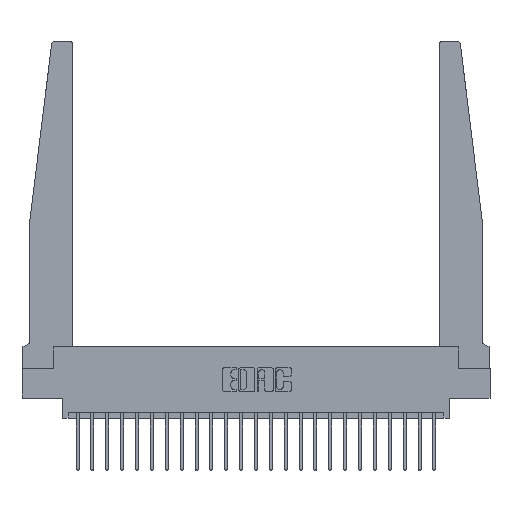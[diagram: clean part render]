
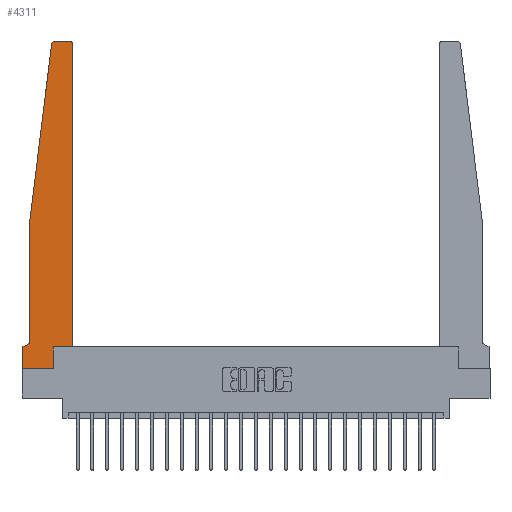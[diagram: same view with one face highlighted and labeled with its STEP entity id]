
A CAD part, top view. The second image highlights one B-rep face of the part: STEP entity #4311.
In plain terms, the highlighted planar face has unit normal (0, 0, 1).
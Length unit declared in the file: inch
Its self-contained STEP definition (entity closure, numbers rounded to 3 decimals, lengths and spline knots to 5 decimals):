
#59 = VERTEX_POINT ( 'NONE', #22046 ) ;
#147 = CARTESIAN_POINT ( 'NONE',  ( 0., 0., 0.37 ) ) ;
#385 = VECTOR ( 'NONE', #1121, 39.37008 ) ;
#510 = CARTESIAN_POINT ( 'NONE',  ( 0., 0.1875, 0.37 ) ) ;
#594 = CIRCLE ( 'NONE', #5047, 0.05 ) ;
#665 = CARTESIAN_POINT ( 'NONE',  ( 0.425, 0.18, 0.37 ) ) ;
#857 = CARTESIAN_POINT ( 'NONE',  ( 0., 0., 0.37 ) ) ;
#860 = LINE ( 'NONE', #13269, #14882 ) ;
#874 = AXIS2_PLACEMENT_3D ( 'NONE', #9341, #22089, #11198 ) ;
#892 = CARTESIAN_POINT ( 'NONE',  ( 0.24675, 2.72367, 0.37 ) ) ;
#988 = CARTESIAN_POINT ( 'NONE',  ( 0.25, 2.75, 0.37 ) ) ;
#1107 = DIRECTION ( 'NONE',  ( 0., 0., -1. ) ) ;
#1121 = DIRECTION ( 'NONE',  ( -1., 0., 0. ) ) ;
#1169 = DIRECTION ( 'NONE',  ( -0.122, -0.992, 0. ) ) ;
#2111 = EDGE_CURVE ( 'NONE', #6656, #59, #3612, .T. ) ;
#2179 = ORIENTED_EDGE ( 'NONE', *, *, #13527, .T. ) ;
#2462 = DIRECTION ( 'NONE',  ( 1., 0., 0. ) ) ;
#2829 = ORIENTED_EDGE ( 'NONE', *, *, #20193, .T. ) ;
#3406 = DIRECTION ( 'NONE',  ( 0., -1., 0. ) ) ;
#3612 = LINE ( 'NONE', #16881, #12784 ) ;
#3784 = CARTESIAN_POINT ( 'NONE',  ( 0.425, 2.72, 0.37 ) ) ;
#4311 = ADVANCED_FACE ( 'NONE', ( #18955 ), #8320, .T. ) ;
#4399 = LINE ( 'NONE', #10229, #13572 ) ;
#4534 = LINE ( 'NONE', #665, #18586 ) ;
#4621 = VERTEX_POINT ( 'NONE', #9284 ) ;
#4689 = CARTESIAN_POINT ( 'NONE',  ( 0., 0.1875, 0.37 ) ) ;
#4871 = VERTEX_POINT ( 'NONE', #857 ) ;
#4925 = LINE ( 'NONE', #21740, #14113 ) ;
#5047 = AXIS2_PLACEMENT_3D ( 'NONE', #12007, #1107, #13897 ) ;
#5271 = VERTEX_POINT ( 'NONE', #7310 ) ;
#5680 = DIRECTION ( 'NONE',  ( 1., 0., 0. ) ) ;
#5751 = LINE ( 'NONE', #10177, #385 ) ;
#5946 = DIRECTION ( 'NONE',  ( 0., 1., 0. ) ) ;
#6105 = VERTEX_POINT ( 'NONE', #7841 ) ;
#6249 = EDGE_CURVE ( 'NONE', #14112, #13678, #5751, .T. ) ;
#6656 = VERTEX_POINT ( 'NONE', #20391 ) ;
#7025 = LINE ( 'NONE', #147, #21035 ) ;
#7199 = DIRECTION ( 'NONE',  ( 0., 1., 0. ) ) ;
#7310 = CARTESIAN_POINT ( 'NONE',  ( 0.2605, 0.18, 0.37 ) ) ;
#7724 = EDGE_CURVE ( 'NONE', #6105, #10409, #860, .T. ) ;
#7751 = EDGE_CURVE ( 'NONE', #5271, #6105, #4534, .T. ) ;
#7841 = CARTESIAN_POINT ( 'NONE',  ( 0.425, 0.18, 0.37 ) ) ;
#8001 = ORIENTED_EDGE ( 'NONE', *, *, #6249, .T. ) ;
#8141 = EDGE_LOOP ( 'NONE', ( #11817, #2829, #23317, #9122, #10008, #8001, #9339, #14277, #2179, #15815, #9830, #22491 ) ) ;
#8252 = DIRECTION ( 'NONE',  ( -1., 0., 0. ) ) ;
#8320 = PLANE ( 'NONE',  #14948 ) ;
#8747 = CARTESIAN_POINT ( 'NONE',  ( 0.395, 2.75, 0.37 ) ) ;
#9122 = ORIENTED_EDGE ( 'NONE', *, *, #2111, .T. ) ;
#9205 = CARTESIAN_POINT ( 'NONE',  ( 0.015, 0.1875, 0.37 ) ) ;
#9284 = CARTESIAN_POINT ( 'NONE',  ( 0.27653, 2.75, 0.37 ) ) ;
#9302 = LINE ( 'NONE', #988, #18513 ) ;
#9339 = ORIENTED_EDGE ( 'NONE', *, *, #20841, .T. ) ;
#9341 = CARTESIAN_POINT ( 'NONE',  ( 0.395, 2.72, 0.37 ) ) ;
#9607 = VECTOR ( 'NONE', #3406, 39.37008 ) ;
#9830 = ORIENTED_EDGE ( 'NONE', *, *, #7724, .T. ) ;
#10008 = ORIENTED_EDGE ( 'NONE', *, *, #19474, .T. ) ;
#10177 = CARTESIAN_POINT ( 'NONE',  ( 0.065, 0.1875, 0.37 ) ) ;
#10178 = LINE ( 'NONE', #12522, #9607 ) ;
#10187 = DIRECTION ( 'NONE',  ( 0., 0., 1. ) ) ;
#10229 = CARTESIAN_POINT ( 'NONE',  ( 0.065, 1.25, 0.37 ) ) ;
#10409 = VERTEX_POINT ( 'NONE', #3784 ) ;
#10447 = EDGE_CURVE ( 'NONE', #4871, #18721, #7025, .T. ) ;
#10551 = DIRECTION ( 'NONE',  ( 0., 0., 1. ) ) ;
#11198 = DIRECTION ( 'NONE',  ( 1., 0., 0. ) ) ;
#11214 = EDGE_CURVE ( 'NONE', #16050, #4621, #9302, .T. ) ;
#11817 = ORIENTED_EDGE ( 'NONE', *, *, #11214, .T. ) ;
#12007 = CARTESIAN_POINT ( 'NONE',  ( 0.015, 0.2375, 0.37 ) ) ;
#12522 = CARTESIAN_POINT ( 'NONE',  ( 0., 0., 0.37 ) ) ;
#12601 = EDGE_CURVE ( 'NONE', #18944, #6656, #4399, .T. ) ;
#12784 = VECTOR ( 'NONE', #18708, 39.37008 ) ;
#13269 = CARTESIAN_POINT ( 'NONE',  ( 0.425, 0.18, 0.37 ) ) ;
#13527 = EDGE_CURVE ( 'NONE', #18721, #5271, #4925, .T. ) ;
#13572 = VECTOR ( 'NONE', #1169, 39.37008 ) ;
#13678 = VERTEX_POINT ( 'NONE', #510 ) ;
#13897 = DIRECTION ( 'NONE',  ( -1., 0., 0. ) ) ;
#14112 = VERTEX_POINT ( 'NONE', #9205 ) ;
#14113 = VECTOR ( 'NONE', #7199, 39.37008 ) ;
#14277 = ORIENTED_EDGE ( 'NONE', *, *, #10447, .T. ) ;
#14806 = EDGE_CURVE ( 'NONE', #10409, #16050, #19429, .T. ) ;
#14882 = VECTOR ( 'NONE', #5946, 39.37008 ) ;
#14948 = AXIS2_PLACEMENT_3D ( 'NONE', #4689, #10187, #22917 ) ;
#15815 = ORIENTED_EDGE ( 'NONE', *, *, #7751, .T. ) ;
#16050 = VERTEX_POINT ( 'NONE', #8747 ) ;
#16737 = CARTESIAN_POINT ( 'NONE',  ( 0.2605, 0., 0.37 ) ) ;
#16881 = CARTESIAN_POINT ( 'NONE',  ( 0.065, 1.25, 0.37 ) ) ;
#18513 = VECTOR ( 'NONE', #8252, 39.37008 ) ;
#18586 = VECTOR ( 'NONE', #2462, 39.37008 ) ;
#18708 = DIRECTION ( 'NONE',  ( 0., -1., 0. ) ) ;
#18721 = VERTEX_POINT ( 'NONE', #16737 ) ;
#18944 = VERTEX_POINT ( 'NONE', #892 ) ;
#18955 = FACE_OUTER_BOUND ( 'NONE', #8141, .T. ) ;
#19429 = CIRCLE ( 'NONE', #874, 0.03 ) ;
#19474 = EDGE_CURVE ( 'NONE', #59, #14112, #594, .T. ) ;
#20193 = EDGE_CURVE ( 'NONE', #4621, #18944, #22736, .T. ) ;
#20391 = CARTESIAN_POINT ( 'NONE',  ( 0.065, 1.25, 0.37 ) ) ;
#20841 = EDGE_CURVE ( 'NONE', #13678, #4871, #10178, .T. ) ;
#21035 = VECTOR ( 'NONE', #5680, 39.37008 ) ;
#21445 = CARTESIAN_POINT ( 'NONE',  ( 0.27653, 2.72, 0.37 ) ) ;
#21740 = CARTESIAN_POINT ( 'NONE',  ( 0.2605, 0.18, 0.37 ) ) ;
#22046 = CARTESIAN_POINT ( 'NONE',  ( 0.065, 0.2375, 0.37 ) ) ;
#22089 = DIRECTION ( 'NONE',  ( 0., 0., 1. ) ) ;
#22491 = ORIENTED_EDGE ( 'NONE', *, *, #14806, .T. ) ;
#22736 = CIRCLE ( 'NONE', #22906, 0.03 ) ;
#22906 = AXIS2_PLACEMENT_3D ( 'NONE', #21445, #10551, #23248 ) ;
#22917 = DIRECTION ( 'NONE',  ( 1., 0., 0. ) ) ;
#23248 = DIRECTION ( 'NONE',  ( 1., 0., 0. ) ) ;
#23317 = ORIENTED_EDGE ( 'NONE', *, *, #12601, .T. ) ;
